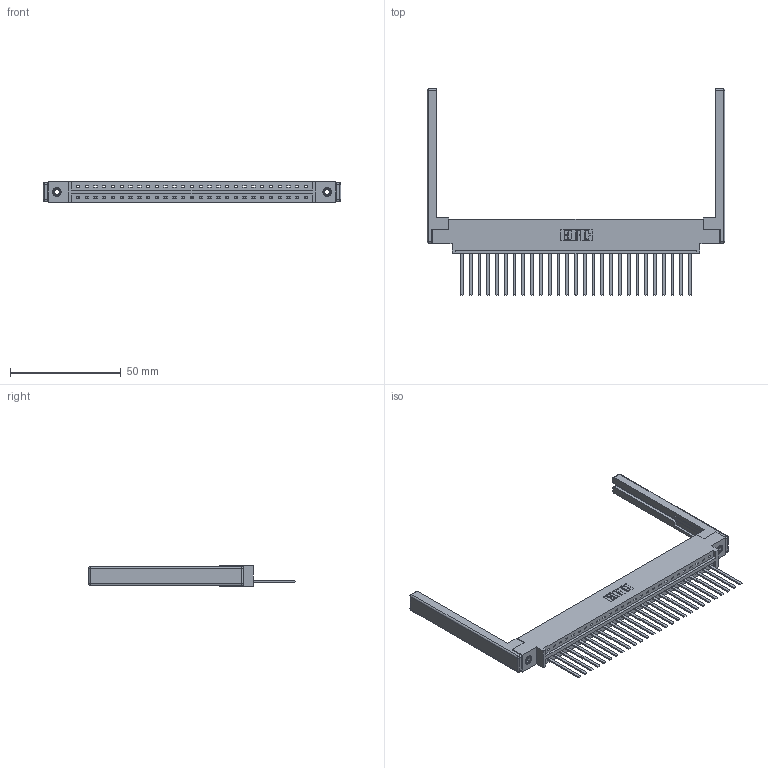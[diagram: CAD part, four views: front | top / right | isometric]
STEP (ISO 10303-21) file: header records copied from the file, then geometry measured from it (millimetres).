
FILE_DESCRIPTION (( 'STEP AP203' ), '1' );
FILE_NAME ('387-027-544-668.STEP', '2019-10-03T14:19:19', ( '' ), ( '' ), 'SwSTEP 2.0', 'SolidWorks 2016', '' );
FILE_SCHEMA (( 'CONFIG_CONTROL_DESIGN' ));
Length unit declared in the file: inch
Products named in the file (5): 337 Part_0.170 Offset - 0.156 Dia-TI; 307-220-068; 345-292-001_345-293-144; 345-250-001_345-250-001-102; 387-027-544-668
Assembly tree (32 placements, depth 2):
  387-027-544-668
    337 Part_0.170 Offset - 0.156 Dia-TI
    345-292-001_345-293-144  x27
    345-250-001_345-250-001-102  x2
    307-220-068  x2
Bounding box: 134.42 x 93.35 x 9.4 mm (x, y, z)
Volume: 18369.1 mm3; surface area: 19578.5 mm2
Topology: 32 solids, 32 shells, 1784 faces, 5303 edges, 3478 vertices
Faces by surface type: plane 1296, cylinder 464, cone 12, sphere 8, torus 4
Entity records: 24718 total; most frequent: CARTESIAN_POINT 4260, ORIENTED_EDGE 4212, DIRECTION 3686, EDGE_CURVE 2106, VECTOR 1932, LINE 1932, VERTEX_POINT 1394, AXIS2_PLACEMENT_3D 877
